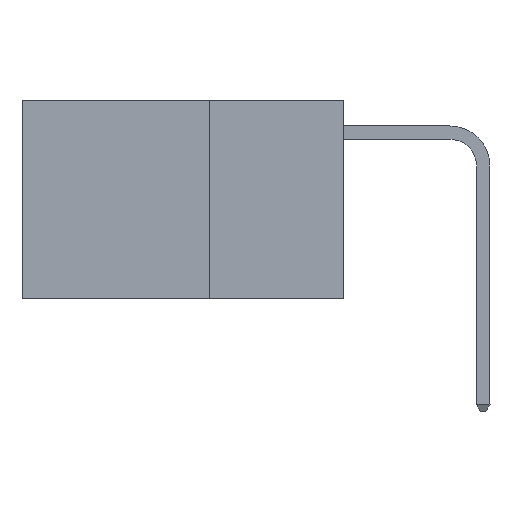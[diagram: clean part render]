
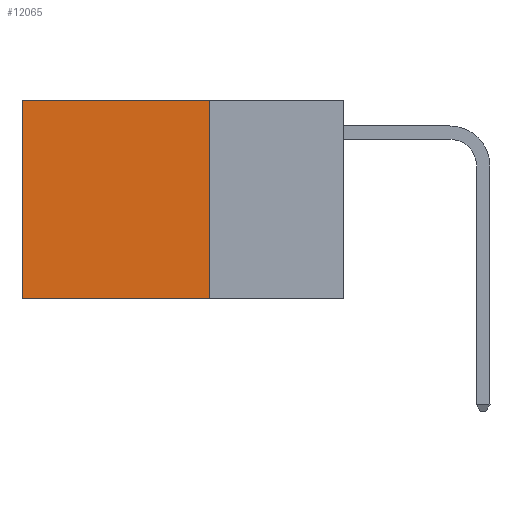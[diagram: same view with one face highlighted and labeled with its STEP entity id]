
A CAD part, left-side view. The second image highlights one B-rep face of the part: STEP entity #12065.
In plain terms, the highlighted planar face has unit normal (-1, 0, 0).
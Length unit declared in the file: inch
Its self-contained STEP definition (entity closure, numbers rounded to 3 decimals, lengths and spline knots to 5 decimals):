
#88 = DIRECTION ( 'NONE',  ( 0., 1., 0. ) ) ;
#382 = LINE ( 'NONE', #3003, #14142 ) ;
#592 = AXIS2_PLACEMENT_3D ( 'NONE', #13135, #1968, #11959 ) ;
#609 = CARTESIAN_POINT ( 'NONE',  ( 0.2625, 0.6, 0. ) ) ;
#1968 = DIRECTION ( 'NONE',  ( 1., 0., 0. ) ) ;
#2382 = CARTESIAN_POINT ( 'NONE',  ( 0.2625, 0.25, 0. ) ) ;
#2401 = CARTESIAN_POINT ( 'NONE',  ( 0.2625, 0.25, -0.37 ) ) ;
#2620 = VECTOR ( 'NONE', #17220, 39.37008 ) ;
#2751 = CARTESIAN_POINT ( 'NONE',  ( 0.2625, 0.6, 0. ) ) ;
#2942 = ORIENTED_EDGE ( 'NONE', *, *, #11709, .F. ) ;
#3003 = CARTESIAN_POINT ( 'NONE',  ( 0.2625, 0.25, 0. ) ) ;
#3671 = LINE ( 'NONE', #609, #10058 ) ;
#5585 = LINE ( 'NONE', #13778, #17595 ) ;
#6985 = VERTEX_POINT ( 'NONE', #2401 ) ;
#7497 = LINE ( 'NONE', #12961, #2620 ) ;
#8041 = CARTESIAN_POINT ( 'NONE',  ( 0.2625, 0.6, -0.37 ) ) ;
#8422 = EDGE_CURVE ( 'NONE', #16293, #9975, #3671, .T. ) ;
#9235 = ORIENTED_EDGE ( 'NONE', *, *, #12142, .F. ) ;
#9764 = ORIENTED_EDGE ( 'NONE', *, *, #12780, .T. ) ;
#9975 = VERTEX_POINT ( 'NONE', #8041 ) ;
#10058 = VECTOR ( 'NONE', #17314, 39.37008 ) ;
#10439 = PLANE ( 'NONE',  #592 ) ;
#11709 = EDGE_CURVE ( 'NONE', #6985, #9975, #5585, .T. ) ;
#11800 = ORIENTED_EDGE ( 'NONE', *, *, #8422, .T. ) ;
#11866 = FACE_OUTER_BOUND ( 'NONE', #15011, .T. ) ;
#11959 = DIRECTION ( 'NONE',  ( 0., 0., -1. ) ) ;
#12065 = ADVANCED_FACE ( 'NONE', ( #11866 ), #10439, .F. ) ;
#12142 = EDGE_CURVE ( 'NONE', #13890, #6985, #7497, .T. ) ;
#12780 = EDGE_CURVE ( 'NONE', #13890, #16293, #382, .T. ) ;
#12961 = CARTESIAN_POINT ( 'NONE',  ( 0.2625, 0.25, 0. ) ) ;
#13135 = CARTESIAN_POINT ( 'NONE',  ( 0.2625, 0.25, 0. ) ) ;
#13778 = CARTESIAN_POINT ( 'NONE',  ( 0.2625, 0.25, -0.37 ) ) ;
#13890 = VERTEX_POINT ( 'NONE', #2382 ) ;
#14086 = DIRECTION ( 'NONE',  ( 0., 1., 0. ) ) ;
#14142 = VECTOR ( 'NONE', #14086, 39.37008 ) ;
#15011 = EDGE_LOOP ( 'NONE', ( #11800, #2942, #9235, #9764 ) ) ;
#16293 = VERTEX_POINT ( 'NONE', #2751 ) ;
#17220 = DIRECTION ( 'NONE',  ( 0., 0., -1. ) ) ;
#17314 = DIRECTION ( 'NONE',  ( 0., 0., -1. ) ) ;
#17595 = VECTOR ( 'NONE', #88, 39.37008 ) ;
